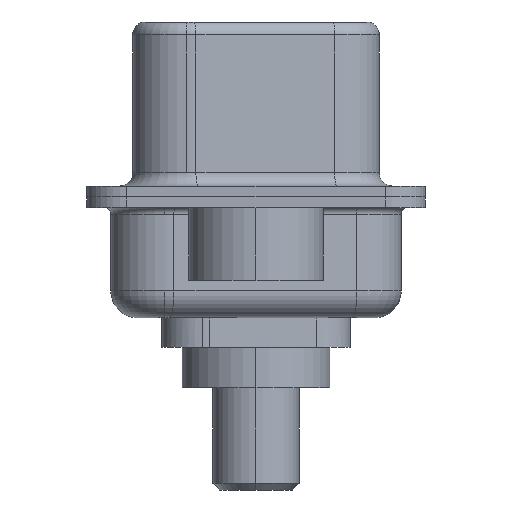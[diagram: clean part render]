
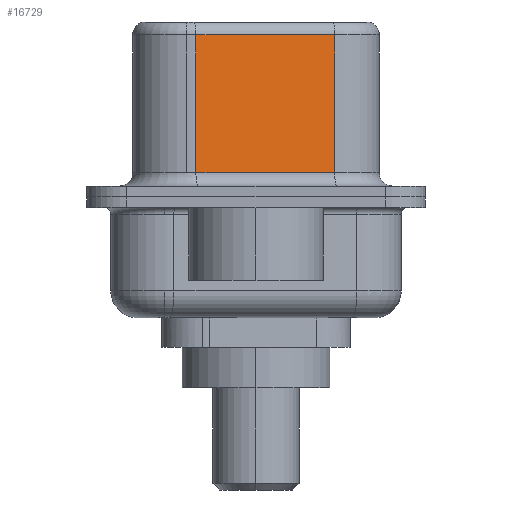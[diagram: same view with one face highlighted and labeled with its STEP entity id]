
A CAD part, left-side view. The second image highlights one B-rep face of the part: STEP entity #16729.
In plain terms, the highlighted planar face has unit normal (-0.985, -0.174, 0).
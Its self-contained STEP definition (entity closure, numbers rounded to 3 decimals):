
#28 = VERTEX_POINT ( 'NONE', #15536 ) ;
#966 = CARTESIAN_POINT ( 'NONE',  ( 4.565, -2.927, 6.02 ) ) ;
#1784 = CARTESIAN_POINT ( 'NONE',  ( 4.565, -2.927, 6.02 ) ) ;
#2078 = LINE ( 'NONE', #9808, #13646 ) ;
#3377 = DIRECTION ( 'NONE',  ( 0.985, 0.174, 0. ) ) ;
#4257 = DIRECTION ( 'NONE',  ( 0., 0., -1. ) ) ;
#5160 = LINE ( 'NONE', #14221, #12055 ) ;
#5641 = CARTESIAN_POINT ( 'NONE',  ( 3.655, 2.233, 6.02 ) ) ;
#5674 = EDGE_CURVE ( 'NONE', #8524, #11630, #8047, .T. ) ;
#6175 = PLANE ( 'NONE',  #15852 ) ;
#6733 = VECTOR ( 'NONE', #8802, 1000. ) ;
#7945 = EDGE_LOOP ( 'NONE', ( #10277, #11649, #9850, #17701 ) ) ;
#8047 = LINE ( 'NONE', #1784, #17864 ) ;
#8497 = VERTEX_POINT ( 'NONE', #15184 ) ;
#8524 = VERTEX_POINT ( 'NONE', #966 ) ;
#8802 = DIRECTION ( 'NONE',  ( 0.174, -0.985, 0. ) ) ;
#9808 = CARTESIAN_POINT ( 'NONE',  ( 3.655, 2.233, 6.52 ) ) ;
#9850 = ORIENTED_EDGE ( 'NONE', *, *, #15152, .T. ) ;
#10277 = ORIENTED_EDGE ( 'NONE', *, *, #10997, .F. ) ;
#10720 = LINE ( 'NONE', #14451, #6733 ) ;
#10997 = EDGE_CURVE ( 'NONE', #8524, #8497, #5160, .T. ) ;
#11056 = EDGE_CURVE ( 'NONE', #28, #8497, #10720, .T. ) ;
#11485 = FACE_OUTER_BOUND ( 'NONE', #7945, .T. ) ;
#11630 = VERTEX_POINT ( 'NONE', #5641 ) ;
#11649 = ORIENTED_EDGE ( 'NONE', *, *, #5674, .T. ) ;
#12055 = VECTOR ( 'NONE', #4257, 1000. ) ;
#12197 = CARTESIAN_POINT ( 'NONE',  ( 4.565, -2.927, 6.52 ) ) ;
#13558 = DIRECTION ( 'NONE',  ( -0.174, 0.985, 0. ) ) ;
#13646 = VECTOR ( 'NONE', #18054, 1000. ) ;
#14221 = CARTESIAN_POINT ( 'NONE',  ( 4.565, -2.927, 6.52 ) ) ;
#14451 = CARTESIAN_POINT ( 'NONE',  ( 4.565, -2.927, 0.9 ) ) ;
#15152 = EDGE_CURVE ( 'NONE', #11630, #28, #2078, .T. ) ;
#15184 = CARTESIAN_POINT ( 'NONE',  ( 4.565, -2.927, 0.9 ) ) ;
#15536 = CARTESIAN_POINT ( 'NONE',  ( 3.655, 2.233, 0.9 ) ) ;
#15852 = AXIS2_PLACEMENT_3D ( 'NONE', #12197, #3377, #13558 ) ;
#16729 = ADVANCED_FACE ( 'NONE', ( #11485 ), #6175, .F. ) ;
#17701 = ORIENTED_EDGE ( 'NONE', *, *, #11056, .T. ) ;
#17741 = DIRECTION ( 'NONE',  ( -0.174, 0.985, 0. ) ) ;
#17864 = VECTOR ( 'NONE', #17741, 1000. ) ;
#18054 = DIRECTION ( 'NONE',  ( 0., 0., -1. ) ) ;
